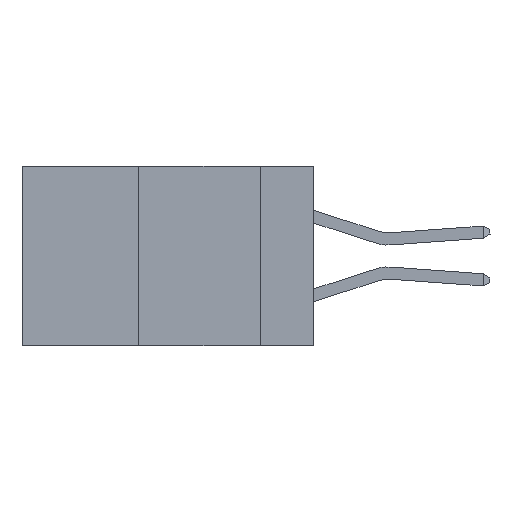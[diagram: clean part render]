
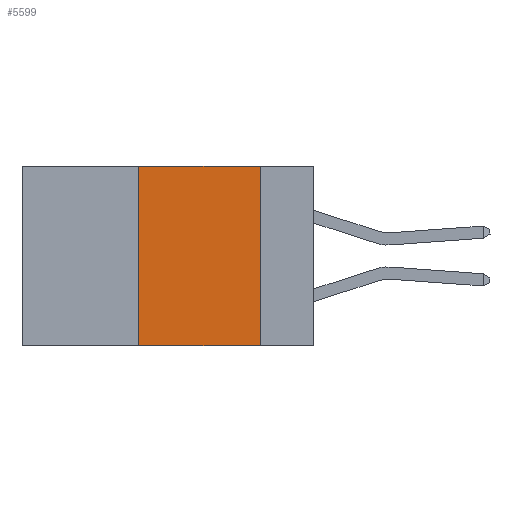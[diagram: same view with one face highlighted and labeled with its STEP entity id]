
A CAD part, left-side view. The second image highlights one B-rep face of the part: STEP entity #5599.
In plain terms, the highlighted planar face has unit normal (-1, 0, 0).
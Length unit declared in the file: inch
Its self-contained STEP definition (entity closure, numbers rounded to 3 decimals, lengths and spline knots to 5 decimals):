
#84 = ORIENTED_EDGE ( 'NONE', *, *, #6973, .T. ) ;
#574 = LINE ( 'NONE', #4104, #4046 ) ;
#736 = LINE ( 'NONE', #7842, #8764 ) ;
#1241 = EDGE_CURVE ( 'NONE', #5252, #3488, #736, .T. ) ;
#1550 = ORIENTED_EDGE ( 'NONE', *, *, #9021, .F. ) ;
#1569 = PLANE ( 'NONE',  #10861 ) ;
#1737 = DIRECTION ( 'NONE',  ( 0., -1., 0. ) ) ;
#2317 = VECTOR ( 'NONE', #1737, 39.37008 ) ;
#2358 = CARTESIAN_POINT ( 'NONE',  ( 0., 0.11, 0. ) ) ;
#2718 = LINE ( 'NONE', #8039, #7927 ) ;
#3488 = VERTEX_POINT ( 'NONE', #8578 ) ;
#4046 = VECTOR ( 'NONE', #7666, 39.37008 ) ;
#4104 = CARTESIAN_POINT ( 'NONE',  ( 0., 0.6, 0. ) ) ;
#5107 = CARTESIAN_POINT ( 'NONE',  ( 0., 0.11, -0.37 ) ) ;
#5252 = VERTEX_POINT ( 'NONE', #10036 ) ;
#5599 = ADVANCED_FACE ( 'NONE', ( #5950 ), #1569, .F. ) ;
#5677 = ORIENTED_EDGE ( 'NONE', *, *, #1241, .F. ) ;
#5950 = FACE_OUTER_BOUND ( 'NONE', #6846, .T. ) ;
#6368 = DIRECTION ( 'NONE',  ( 0., 0., 1. ) ) ;
#6641 = ORIENTED_EDGE ( 'NONE', *, *, #7079, .F. ) ;
#6846 = EDGE_LOOP ( 'NONE', ( #6641, #1550, #5677, #84 ) ) ;
#6973 = EDGE_CURVE ( 'NONE', #5252, #7762, #9901, .T. ) ;
#7079 = EDGE_CURVE ( 'NONE', #9067, #7762, #2718, .T. ) ;
#7109 = DIRECTION ( 'NONE',  ( 0., 0., -1. ) ) ;
#7666 = DIRECTION ( 'NONE',  ( 0., -1., 0. ) ) ;
#7753 = DIRECTION ( 'NONE',  ( 0., 0., -1. ) ) ;
#7762 = VERTEX_POINT ( 'NONE', #5107 ) ;
#7842 = CARTESIAN_POINT ( 'NONE',  ( 0., 0.36, 0. ) ) ;
#7927 = VECTOR ( 'NONE', #7109, 39.37008 ) ;
#8039 = CARTESIAN_POINT ( 'NONE',  ( 0., 0.11, 0. ) ) ;
#8498 = CARTESIAN_POINT ( 'NONE',  ( 0., 0.6, 0. ) ) ;
#8578 = CARTESIAN_POINT ( 'NONE',  ( 0., 0.36, 0. ) ) ;
#8764 = VECTOR ( 'NONE', #6368, 39.37008 ) ;
#9021 = EDGE_CURVE ( 'NONE', #3488, #9067, #574, .T. ) ;
#9067 = VERTEX_POINT ( 'NONE', #2358 ) ;
#9901 = LINE ( 'NONE', #10554, #2317 ) ;
#10036 = CARTESIAN_POINT ( 'NONE',  ( 0., 0.36, -0.37 ) ) ;
#10257 = DIRECTION ( 'NONE',  ( 1., 0., 0. ) ) ;
#10554 = CARTESIAN_POINT ( 'NONE',  ( 0., 0.6, -0.37 ) ) ;
#10861 = AXIS2_PLACEMENT_3D ( 'NONE', #8498, #10257, #7753 ) ;
